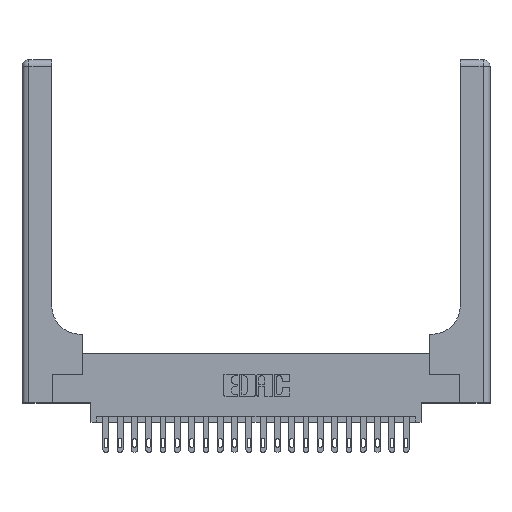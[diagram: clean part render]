
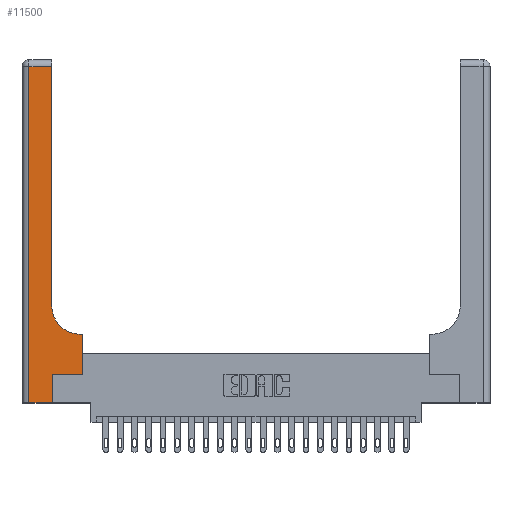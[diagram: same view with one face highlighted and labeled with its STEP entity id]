
A CAD part, top view. The second image highlights one B-rep face of the part: STEP entity #11500.
In plain terms, the highlighted planar face has unit normal (0, 0, 1).
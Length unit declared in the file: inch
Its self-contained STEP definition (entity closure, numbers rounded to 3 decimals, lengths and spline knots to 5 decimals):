
#129 = DIRECTION ( 'NONE',  ( 0., -1., 0. ) ) ;
#241 = CARTESIAN_POINT ( 'NONE',  ( 0.06, 2.94, 0.37 ) ) ;
#788 = ORIENTED_EDGE ( 'NONE', *, *, #885, .T. ) ;
#792 = ORIENTED_EDGE ( 'NONE', *, *, #13845, .T. ) ;
#808 = LINE ( 'NONE', #21862, #15417 ) ;
#862 = VECTOR ( 'NONE', #2485, 39.37008 ) ;
#885 = EDGE_CURVE ( 'NONE', #16604, #13099, #11216, .T. ) ;
#1055 = LINE ( 'NONE', #8081, #21800 ) ;
#1467 = EDGE_CURVE ( 'NONE', #16513, #21806, #14979, .T. ) ;
#2284 = EDGE_CURVE ( 'NONE', #8134, #10639, #18397, .T. ) ;
#2485 = DIRECTION ( 'NONE',  ( 0., 1., 0. ) ) ;
#2639 = ORIENTED_EDGE ( 'NONE', *, *, #16915, .T. ) ;
#2714 = DIRECTION ( 'NONE',  ( 0., 0., -1. ) ) ;
#2755 = LINE ( 'NONE', #14724, #3305 ) ;
#2830 = CARTESIAN_POINT ( 'NONE',  ( 0.51, 0.85, 0.37 ) ) ;
#2845 = VERTEX_POINT ( 'NONE', #241 ) ;
#3305 = VECTOR ( 'NONE', #6435, 39.37008 ) ;
#4994 = DIRECTION ( 'NONE',  ( 0., 0., -1. ) ) ;
#5114 = AXIS2_PLACEMENT_3D ( 'NONE', #17315, #4994, #20988 ) ;
#5989 = VERTEX_POINT ( 'NONE', #13995 ) ;
#6354 = DIRECTION ( 'NONE',  ( -1., 0., 0. ) ) ;
#6435 = DIRECTION ( 'NONE',  ( 0., 1., 0. ) ) ;
#6763 = EDGE_CURVE ( 'NONE', #10639, #16604, #808, .T. ) ;
#7488 = CARTESIAN_POINT ( 'NONE',  ( 0.51, 0.6, 0.37 ) ) ;
#7657 = DIRECTION ( 'NONE',  ( 1., 0., 0. ) ) ;
#7690 = CARTESIAN_POINT ( 'NONE',  ( 0., 0., 0.37 ) ) ;
#7856 = CARTESIAN_POINT ( 'NONE',  ( 0.26, 0.6, 0.37 ) ) ;
#8081 = CARTESIAN_POINT ( 'NONE',  ( 0., 2.94, 0.37 ) ) ;
#8134 = VERTEX_POINT ( 'NONE', #18461 ) ;
#8278 = EDGE_CURVE ( 'NONE', #13099, #16513, #2755, .T. ) ;
#9844 = DIRECTION ( 'NONE',  ( 1., 0., 0. ) ) ;
#10167 = FACE_OUTER_BOUND ( 'NONE', #13029, .T. ) ;
#10272 = LINE ( 'NONE', #17308, #22227 ) ;
#10555 = CARTESIAN_POINT ( 'NONE',  ( 0.265, 0.25, 0.37 ) ) ;
#10639 = VERTEX_POINT ( 'NONE', #13699 ) ;
#11069 = ORIENTED_EDGE ( 'NONE', *, *, #6763, .T. ) ;
#11206 = ORIENTED_EDGE ( 'NONE', *, *, #11865, .T. ) ;
#11216 = LINE ( 'NONE', #12597, #18969 ) ;
#11500 = ADVANCED_FACE ( 'NONE', ( #10167 ), #20753, .F. ) ;
#11557 = CARTESIAN_POINT ( 'NONE',  ( 0.26, 3., 0.37 ) ) ;
#11865 = EDGE_CURVE ( 'NONE', #15262, #2845, #1055, .T. ) ;
#12019 = ORIENTED_EDGE ( 'NONE', *, *, #15776, .T. ) ;
#12597 = CARTESIAN_POINT ( 'NONE',  ( 0.265, 0.25, 0.37 ) ) ;
#13029 = EDGE_LOOP ( 'NONE', ( #792, #11206, #12019, #13219, #11069, #788, #18247, #19888, #2639 ) ) ;
#13099 = VERTEX_POINT ( 'NONE', #20599 ) ;
#13219 = ORIENTED_EDGE ( 'NONE', *, *, #2284, .T. ) ;
#13699 = CARTESIAN_POINT ( 'NONE',  ( 0.265, 0., 0.37 ) ) ;
#13845 = EDGE_CURVE ( 'NONE', #5989, #15262, #18484, .T. ) ;
#13995 = CARTESIAN_POINT ( 'NONE',  ( 0.26, 0.85, 0.37 ) ) ;
#14724 = CARTESIAN_POINT ( 'NONE',  ( 0.528, 0.25, 0.37 ) ) ;
#14865 = DIRECTION ( 'NONE',  ( -1., 0., 0. ) ) ;
#14979 = LINE ( 'NONE', #7856, #21924 ) ;
#15044 = CARTESIAN_POINT ( 'NONE',  ( 0.528, 0.6, 0.37 ) ) ;
#15262 = VERTEX_POINT ( 'NONE', #22607 ) ;
#15417 = VECTOR ( 'NONE', #16925, 39.37008 ) ;
#15776 = EDGE_CURVE ( 'NONE', #2845, #8134, #10272, .T. ) ;
#16513 = VERTEX_POINT ( 'NONE', #15044 ) ;
#16604 = VERTEX_POINT ( 'NONE', #10555 ) ;
#16915 = EDGE_CURVE ( 'NONE', #21806, #5989, #17516, .T. ) ;
#16925 = DIRECTION ( 'NONE',  ( 0., 1., 0. ) ) ;
#17308 = CARTESIAN_POINT ( 'NONE',  ( 0.06, 3., 0.37 ) ) ;
#17315 = CARTESIAN_POINT ( 'NONE',  ( 0., 3., 0.37 ) ) ;
#17516 = CIRCLE ( 'NONE', #22281, 0.25 ) ;
#18247 = ORIENTED_EDGE ( 'NONE', *, *, #8278, .T. ) ;
#18397 = LINE ( 'NONE', #7690, #20628 ) ;
#18461 = CARTESIAN_POINT ( 'NONE',  ( 0.06, 0., 0.37 ) ) ;
#18484 = LINE ( 'NONE', #11557, #862 ) ;
#18969 = VECTOR ( 'NONE', #7657, 39.37008 ) ;
#19888 = ORIENTED_EDGE ( 'NONE', *, *, #1467, .T. ) ;
#20599 = CARTESIAN_POINT ( 'NONE',  ( 0.528, 0.25, 0.37 ) ) ;
#20628 = VECTOR ( 'NONE', #21727, 39.37008 ) ;
#20753 = PLANE ( 'NONE',  #5114 ) ;
#20988 = DIRECTION ( 'NONE',  ( -1., 0., 0. ) ) ;
#21727 = DIRECTION ( 'NONE',  ( 1., 0., 0. ) ) ;
#21800 = VECTOR ( 'NONE', #6354, 39.37008 ) ;
#21806 = VERTEX_POINT ( 'NONE', #7488 ) ;
#21862 = CARTESIAN_POINT ( 'NONE',  ( 0.265, 0., 0.37 ) ) ;
#21924 = VECTOR ( 'NONE', #14865, 39.37008 ) ;
#22227 = VECTOR ( 'NONE', #129, 39.37008 ) ;
#22281 = AXIS2_PLACEMENT_3D ( 'NONE', #2830, #2714, #9844 ) ;
#22607 = CARTESIAN_POINT ( 'NONE',  ( 0.26, 2.94, 0.37 ) ) ;
